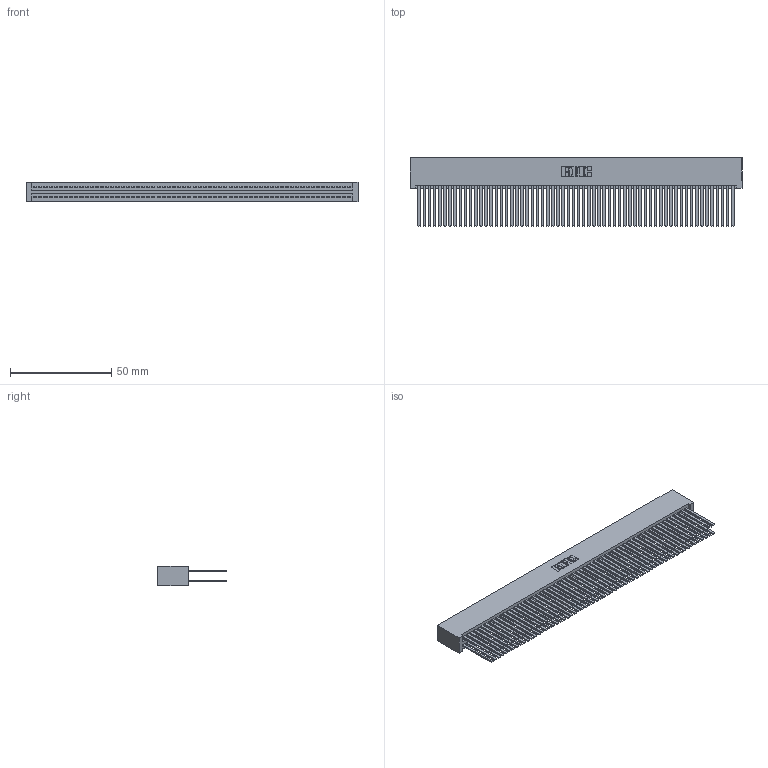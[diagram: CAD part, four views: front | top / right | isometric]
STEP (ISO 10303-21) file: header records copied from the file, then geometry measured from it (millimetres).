
FILE_DESCRIPTION (( 'STEP AP203' ), '1' );
FILE_NAME ('345-124-544-201.STEP', '2018-10-19T10:22:59', ( '' ), ( '' ), 'SwSTEP 2.0', 'SolidWorks 2016', '' );
FILE_SCHEMA (( 'CONFIG_CONTROL_DESIGN' ));
Length unit declared in the file: inch
Products named in the file (3): 345 Part_No Mounting Lugs; 345-292-001_345-293-144; 345-124-544-201
Assembly tree (125 placements, depth 2):
  345-124-544-201
    345 Part_No Mounting Lugs
    345-292-001_345-293-144  x124
Bounding box: 164.08 x 33.96 x 9.4 mm (x, y, z)
Volume: 18479.1 mm3; surface area: 33100.5 mm2
Topology: 125 solids, 125 shells, 5574 faces, 16561 edges, 10874 vertices
Faces by surface type: plane 3672, cylinder 1902
Entity records: 45493 total; most frequent: CARTESIAN_POINT 7604, ORIENTED_EDGE 7538, DIRECTION 6673, EDGE_CURVE 3769, VECTOR 3401, LINE 3401, VERTEX_POINT 2510, AXIS2_PLACEMENT_3D 1636
